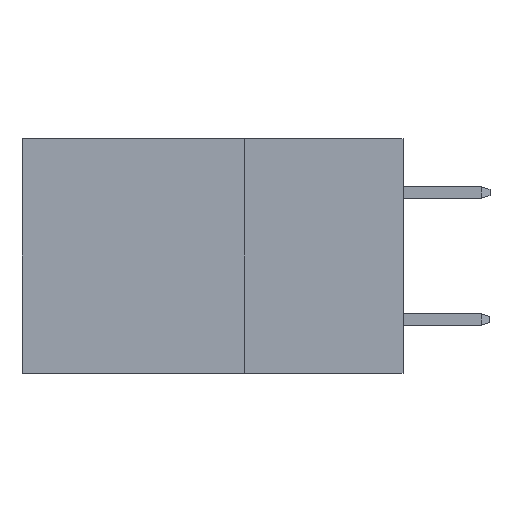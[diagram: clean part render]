
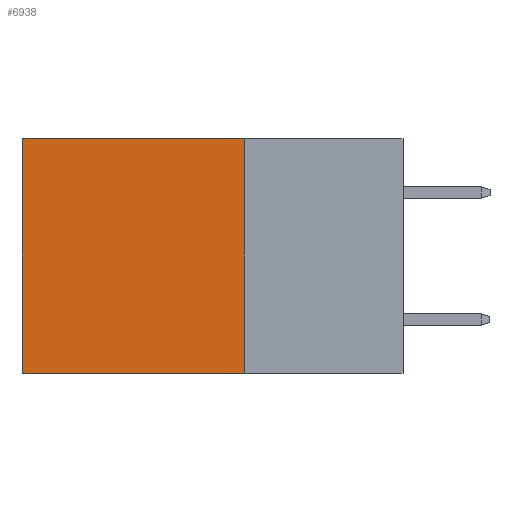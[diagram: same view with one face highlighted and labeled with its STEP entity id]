
A CAD part, left-side view. The second image highlights one B-rep face of the part: STEP entity #6938.
In plain terms, the highlighted planar face has unit normal (-1, 0, 0).
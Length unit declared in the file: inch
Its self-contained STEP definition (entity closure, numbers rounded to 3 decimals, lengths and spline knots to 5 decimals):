
#387 = VERTEX_POINT ( 'NONE', #10822 ) ;
#393 = CARTESIAN_POINT ( 'NONE',  ( 0.2875, 0.25, 0. ) ) ;
#788 = CARTESIAN_POINT ( 'NONE',  ( 0.2875, 0.25, 0. ) ) ;
#1046 = CARTESIAN_POINT ( 'NONE',  ( 0.2875, 0.25, -0.37 ) ) ;
#1306 = VECTOR ( 'NONE', #2149, 39.37008 ) ;
#1604 = DIRECTION ( 'NONE',  ( 0., 0., -1. ) ) ;
#1807 = DIRECTION ( 'NONE',  ( 0., 0., -1. ) ) ;
#2149 = DIRECTION ( 'NONE',  ( 0., 1., 0. ) ) ;
#2803 = PLANE ( 'NONE',  #7812 ) ;
#2929 = CARTESIAN_POINT ( 'NONE',  ( 0.2875, 0.25, 0. ) ) ;
#3161 = LINE ( 'NONE', #788, #11331 ) ;
#3577 = VERTEX_POINT ( 'NONE', #1046 ) ;
#3744 = EDGE_CURVE ( 'NONE', #9501, #3577, #3161, .T. ) ;
#4514 = DIRECTION ( 'NONE',  ( 1., 0., 0. ) ) ;
#4793 = LINE ( 'NONE', #6599, #1306 ) ;
#4867 = VECTOR ( 'NONE', #10306, 39.37008 ) ;
#4959 = ORIENTED_EDGE ( 'NONE', *, *, #11162, .F. ) ;
#5329 = LINE ( 'NONE', #9838, #9781 ) ;
#5494 = CARTESIAN_POINT ( 'NONE',  ( 0.2875, 0.25, 0. ) ) ;
#6599 = CARTESIAN_POINT ( 'NONE',  ( 0.2875, 0.25, -0.37 ) ) ;
#6938 = ADVANCED_FACE ( 'NONE', ( #7249 ), #2803, .F. ) ;
#7032 = EDGE_LOOP ( 'NONE', ( #9014, #4959, #8880, #11180 ) ) ;
#7249 = FACE_OUTER_BOUND ( 'NONE', #7032, .T. ) ;
#7812 = AXIS2_PLACEMENT_3D ( 'NONE', #5494, #4514, #9942 ) ;
#7847 = VERTEX_POINT ( 'NONE', #8745 ) ;
#8259 = LINE ( 'NONE', #2929, #4867 ) ;
#8745 = CARTESIAN_POINT ( 'NONE',  ( 0.2875, 0.6, -0.37 ) ) ;
#8880 = ORIENTED_EDGE ( 'NONE', *, *, #3744, .F. ) ;
#9014 = ORIENTED_EDGE ( 'NONE', *, *, #9717, .T. ) ;
#9501 = VERTEX_POINT ( 'NONE', #393 ) ;
#9717 = EDGE_CURVE ( 'NONE', #387, #7847, #5329, .T. ) ;
#9781 = VECTOR ( 'NONE', #1807, 39.37008 ) ;
#9838 = CARTESIAN_POINT ( 'NONE',  ( 0.2875, 0.6, 0. ) ) ;
#9942 = DIRECTION ( 'NONE',  ( 0., 0., -1. ) ) ;
#10306 = DIRECTION ( 'NONE',  ( 0., 1., 0. ) ) ;
#10732 = EDGE_CURVE ( 'NONE', #9501, #387, #8259, .T. ) ;
#10822 = CARTESIAN_POINT ( 'NONE',  ( 0.2875, 0.6, 0. ) ) ;
#11162 = EDGE_CURVE ( 'NONE', #3577, #7847, #4793, .T. ) ;
#11180 = ORIENTED_EDGE ( 'NONE', *, *, #10732, .T. ) ;
#11331 = VECTOR ( 'NONE', #1604, 39.37008 ) ;
